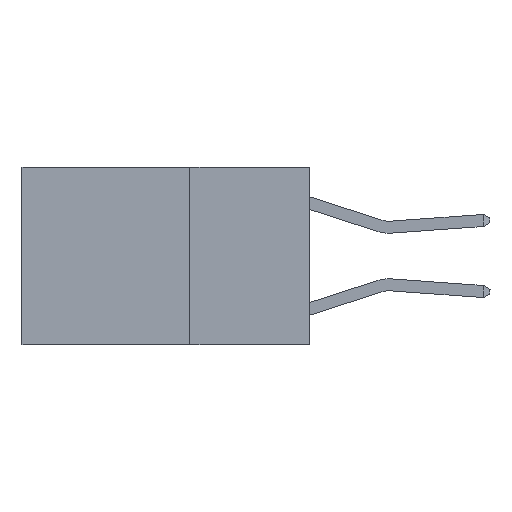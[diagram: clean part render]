
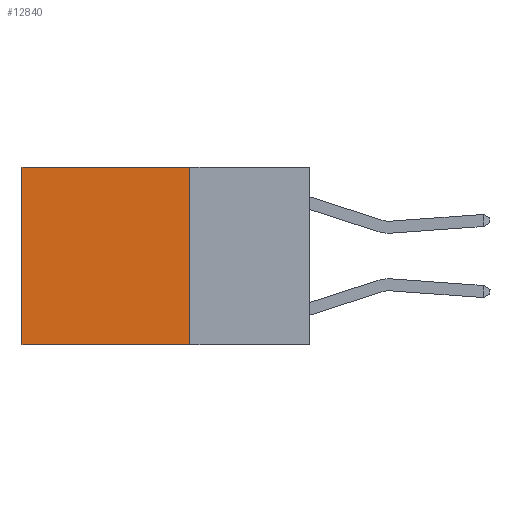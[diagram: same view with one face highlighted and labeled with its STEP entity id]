
A CAD part, left-side view. The second image highlights one B-rep face of the part: STEP entity #12840.
In plain terms, the highlighted planar face has unit normal (-1, 0, 0).
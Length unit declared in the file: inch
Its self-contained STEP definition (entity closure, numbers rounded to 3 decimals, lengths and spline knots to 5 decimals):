
#1222 = ORIENTED_EDGE ( 'NONE', *, *, #20318, .F. ) ;
#2292 = DIRECTION ( 'NONE',  ( 0., 0., -1. ) ) ;
#3424 = VERTEX_POINT ( 'NONE', #16826 ) ;
#4119 = EDGE_CURVE ( 'NONE', #18486, #13705, #13237, .T. ) ;
#4803 = DIRECTION ( 'NONE',  ( 0., 0., -1. ) ) ;
#4905 = EDGE_CURVE ( 'NONE', #3424, #13705, #15133, .T. ) ;
#5128 = DIRECTION ( 'NONE',  ( 0., 1., 0. ) ) ;
#8711 = CARTESIAN_POINT ( 'NONE',  ( 0.2625, 0.25, 0. ) ) ;
#8983 = EDGE_LOOP ( 'NONE', ( #12711, #12968, #1222, #13176 ) ) ;
#10820 = PLANE ( 'NONE',  #12979 ) ;
#10949 = FACE_OUTER_BOUND ( 'NONE', #8983, .T. ) ;
#11871 = DIRECTION ( 'NONE',  ( 0., 1., 0. ) ) ;
#12006 = VERTEX_POINT ( 'NONE', #12998 ) ;
#12711 = ORIENTED_EDGE ( 'NONE', *, *, #4119, .T. ) ;
#12840 = ADVANCED_FACE ( 'NONE', ( #10949 ), #10820, .F. ) ;
#12917 = DIRECTION ( 'NONE',  ( 0., 0., -1. ) ) ;
#12968 = ORIENTED_EDGE ( 'NONE', *, *, #4905, .F. ) ;
#12979 = AXIS2_PLACEMENT_3D ( 'NONE', #8711, #25199, #12917 ) ;
#12998 = CARTESIAN_POINT ( 'NONE',  ( 0.2625, 0.25, 0. ) ) ;
#13176 = ORIENTED_EDGE ( 'NONE', *, *, #15233, .T. ) ;
#13237 = LINE ( 'NONE', #19180, #16783 ) ;
#13705 = VERTEX_POINT ( 'NONE', #23720 ) ;
#15128 = CARTESIAN_POINT ( 'NONE',  ( 0.2625, 0.6, 0. ) ) ;
#15133 = LINE ( 'NONE', #15407, #19920 ) ;
#15233 = EDGE_CURVE ( 'NONE', #12006, #18486, #24634, .T. ) ;
#15407 = CARTESIAN_POINT ( 'NONE',  ( 0.2625, 0.25, -0.37 ) ) ;
#16734 = CARTESIAN_POINT ( 'NONE',  ( 0.2625, 0.25, 0. ) ) ;
#16783 = VECTOR ( 'NONE', #4803, 39.37008 ) ;
#16826 = CARTESIAN_POINT ( 'NONE',  ( 0.2625, 0.25, -0.37 ) ) ;
#18486 = VERTEX_POINT ( 'NONE', #15128 ) ;
#18769 = LINE ( 'NONE', #16734, #24235 ) ;
#19180 = CARTESIAN_POINT ( 'NONE',  ( 0.2625, 0.6, 0. ) ) ;
#19822 = VECTOR ( 'NONE', #11871, 39.37008 ) ;
#19920 = VECTOR ( 'NONE', #5128, 39.37008 ) ;
#20318 = EDGE_CURVE ( 'NONE', #12006, #3424, #18769, .T. ) ;
#23720 = CARTESIAN_POINT ( 'NONE',  ( 0.2625, 0.6, -0.37 ) ) ;
#24174 = CARTESIAN_POINT ( 'NONE',  ( 0.2625, 0.25, 0. ) ) ;
#24235 = VECTOR ( 'NONE', #2292, 39.37008 ) ;
#24634 = LINE ( 'NONE', #24174, #19822 ) ;
#25199 = DIRECTION ( 'NONE',  ( 1., 0., 0. ) ) ;
